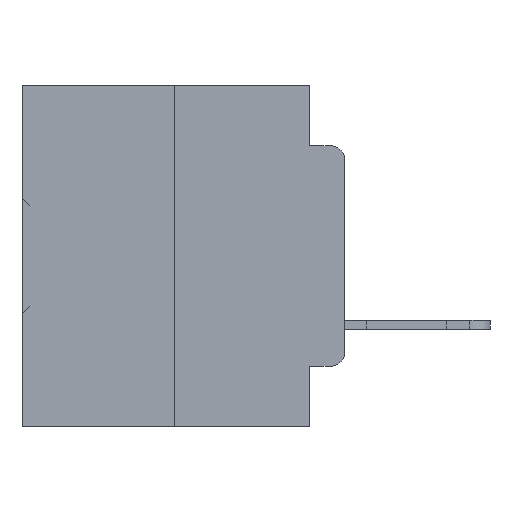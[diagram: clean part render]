
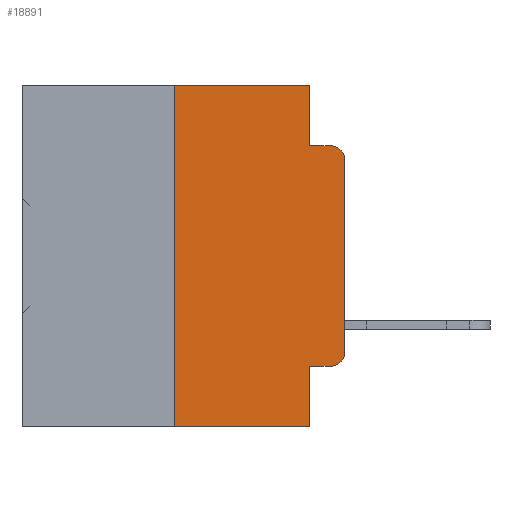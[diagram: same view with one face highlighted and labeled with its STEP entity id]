
A CAD part, left-side view. The second image highlights one B-rep face of the part: STEP entity #18891.
In plain terms, the highlighted planar face has unit normal (-1, 0, 0).
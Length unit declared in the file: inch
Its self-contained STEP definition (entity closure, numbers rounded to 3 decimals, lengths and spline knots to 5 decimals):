
#841 = VECTOR ( 'NONE', #23424, 39.37008 ) ;
#993 = CARTESIAN_POINT ( 'NONE',  ( 0., 0.051, 0. ) ) ;
#1163 = CARTESIAN_POINT ( 'NONE',  ( 0., 0.25, -0.5 ) ) ;
#1237 = VERTEX_POINT ( 'NONE', #37083 ) ;
#1990 = ORIENTED_EDGE ( 'NONE', *, *, #21325, .T. ) ;
#2049 = CARTESIAN_POINT ( 'NONE',  ( 0., 0.051, -0.5 ) ) ;
#3464 = VERTEX_POINT ( 'NONE', #25385 ) ;
#4095 = CARTESIAN_POINT ( 'NONE',  ( 0., 0.02, -0.1085 ) ) ;
#4350 = DIRECTION ( 'NONE',  ( 0., 0., 1. ) ) ;
#4784 = CIRCLE ( 'NONE', #11150, 0.02 ) ;
#5203 = VECTOR ( 'NONE', #4350, 39.37008 ) ;
#5567 = AXIS2_PLACEMENT_3D ( 'NONE', #20689, #20496, #20454 ) ;
#6037 = CIRCLE ( 'NONE', #9103, 0.02 ) ;
#7204 = DIRECTION ( 'NONE',  ( 0., 0., -1. ) ) ;
#7520 = CARTESIAN_POINT ( 'NONE',  ( 0., 0.051, -0.4115 ) ) ;
#8787 = DIRECTION ( 'NONE',  ( 0., -1., 0. ) ) ;
#8899 = VERTEX_POINT ( 'NONE', #27177 ) ;
#9103 = AXIS2_PLACEMENT_3D ( 'NONE', #32313, #15431, #34953 ) ;
#9450 = DIRECTION ( 'NONE',  ( 0., -1., 0. ) ) ;
#10138 = LINE ( 'NONE', #36833, #841 ) ;
#10424 = CARTESIAN_POINT ( 'NONE',  ( 0., 0.25, 0. ) ) ;
#10512 = CARTESIAN_POINT ( 'NONE',  ( 0., 0.473, 0. ) ) ;
#11150 = AXIS2_PLACEMENT_3D ( 'NONE', #4095, #24915, #7204 ) ;
#11944 = CARTESIAN_POINT ( 'NONE',  ( 0., 0., -0.1085 ) ) ;
#12221 = ORIENTED_EDGE ( 'NONE', *, *, #32720, .F. ) ;
#12433 = ORIENTED_EDGE ( 'NONE', *, *, #21309, .F. ) ;
#12943 = VECTOR ( 'NONE', #18624, 39.37008 ) ;
#13971 = LINE ( 'NONE', #7520, #35401 ) ;
#14109 = FACE_OUTER_BOUND ( 'NONE', #22666, .T. ) ;
#15431 = DIRECTION ( 'NONE',  ( -1., 0., 0. ) ) ;
#16595 = ORIENTED_EDGE ( 'NONE', *, *, #32760, .F. ) ;
#17239 = ORIENTED_EDGE ( 'NONE', *, *, #30258, .F. ) ;
#17386 = CARTESIAN_POINT ( 'NONE',  ( 0., 0.051, -0.0885 ) ) ;
#17501 = CARTESIAN_POINT ( 'NONE',  ( 0., 0.051, 0. ) ) ;
#17966 = EDGE_CURVE ( 'NONE', #22388, #25998, #31901, .T. ) ;
#18577 = CARTESIAN_POINT ( 'NONE',  ( 0., 0.02, -0.4115 ) ) ;
#18624 = DIRECTION ( 'NONE',  ( 0., -1., 0. ) ) ;
#18891 = ADVANCED_FACE ( 'NONE', ( #14109 ), #20786, .F. ) ;
#19001 = VERTEX_POINT ( 'NONE', #17386 ) ;
#19031 = CARTESIAN_POINT ( 'NONE',  ( 0., 0.25, 0. ) ) ;
#20199 = LINE ( 'NONE', #10424, #5203 ) ;
#20453 = ORIENTED_EDGE ( 'NONE', *, *, #32453, .F. ) ;
#20454 = DIRECTION ( 'NONE',  ( 0., 0., -1. ) ) ;
#20496 = DIRECTION ( 'NONE',  ( 1., 0., 0. ) ) ;
#20689 = CARTESIAN_POINT ( 'NONE',  ( 0., 0.473, 0. ) ) ;
#20786 = PLANE ( 'NONE',  #5567 ) ;
#20926 = ORIENTED_EDGE ( 'NONE', *, *, #17966, .T. ) ;
#21309 = EDGE_CURVE ( 'NONE', #21931, #3464, #36159, .T. ) ;
#21325 = EDGE_CURVE ( 'NONE', #8899, #25469, #13971, .T. ) ;
#21563 = ORIENTED_EDGE ( 'NONE', *, *, #31725, .T. ) ;
#21931 = VERTEX_POINT ( 'NONE', #19031 ) ;
#22040 = ORIENTED_EDGE ( 'NONE', *, *, #32020, .T. ) ;
#22388 = VERTEX_POINT ( 'NONE', #1163 ) ;
#22666 = EDGE_LOOP ( 'NONE', ( #21563, #22040, #20453, #12221, #12433, #16595, #20926, #17239, #1990, #31332 ) ) ;
#22934 = VECTOR ( 'NONE', #33143, 39.37008 ) ;
#23424 = DIRECTION ( 'NONE',  ( 0., 0., 1. ) ) ;
#24915 = DIRECTION ( 'NONE',  ( -1., 0., 0. ) ) ;
#25385 = CARTESIAN_POINT ( 'NONE',  ( 0., 0.051, 0. ) ) ;
#25469 = VERTEX_POINT ( 'NONE', #18577 ) ;
#25480 = VECTOR ( 'NONE', #32905, 39.37008 ) ;
#25998 = VERTEX_POINT ( 'NONE', #2049 ) ;
#26126 = DIRECTION ( 'NONE',  ( 0., 0., -1. ) ) ;
#27177 = CARTESIAN_POINT ( 'NONE',  ( 0., 0.051, -0.4115 ) ) ;
#27525 = VECTOR ( 'NONE', #26126, 39.37008 ) ;
#28074 = VERTEX_POINT ( 'NONE', #29595 ) ;
#28642 = LINE ( 'NONE', #993, #22934 ) ;
#29088 = LINE ( 'NONE', #29837, #12943 ) ;
#29595 = CARTESIAN_POINT ( 'NONE',  ( 0., 0.02, -0.0885 ) ) ;
#29635 = VERTEX_POINT ( 'NONE', #11944 ) ;
#29837 = CARTESIAN_POINT ( 'NONE',  ( 0., 0.051, -0.0885 ) ) ;
#30019 = VECTOR ( 'NONE', #9450, 39.37008 ) ;
#30258 = EDGE_CURVE ( 'NONE', #8899, #25998, #34709, .T. ) ;
#31332 = ORIENTED_EDGE ( 'NONE', *, *, #35222, .T. ) ;
#31725 = EDGE_CURVE ( 'NONE', #1237, #29635, #10138, .T. ) ;
#31901 = LINE ( 'NONE', #33017, #25480 ) ;
#32020 = EDGE_CURVE ( 'NONE', #29635, #28074, #4784, .T. ) ;
#32313 = CARTESIAN_POINT ( 'NONE',  ( 0., 0.02, -0.3915 ) ) ;
#32453 = EDGE_CURVE ( 'NONE', #19001, #28074, #29088, .T. ) ;
#32720 = EDGE_CURVE ( 'NONE', #3464, #19001, #28642, .T. ) ;
#32760 = EDGE_CURVE ( 'NONE', #22388, #21931, #20199, .T. ) ;
#32905 = DIRECTION ( 'NONE',  ( 0., -1., 0. ) ) ;
#33017 = CARTESIAN_POINT ( 'NONE',  ( 0., 0.473, -0.5 ) ) ;
#33143 = DIRECTION ( 'NONE',  ( 0., 0., -1. ) ) ;
#34709 = LINE ( 'NONE', #17501, #27525 ) ;
#34953 = DIRECTION ( 'NONE',  ( 0., 0., -1. ) ) ;
#35222 = EDGE_CURVE ( 'NONE', #25469, #1237, #6037, .T. ) ;
#35401 = VECTOR ( 'NONE', #8787, 39.37008 ) ;
#36159 = LINE ( 'NONE', #10512, #30019 ) ;
#36833 = CARTESIAN_POINT ( 'NONE',  ( 0., 0., 0. ) ) ;
#37083 = CARTESIAN_POINT ( 'NONE',  ( 0., 0., -0.3915 ) ) ;
